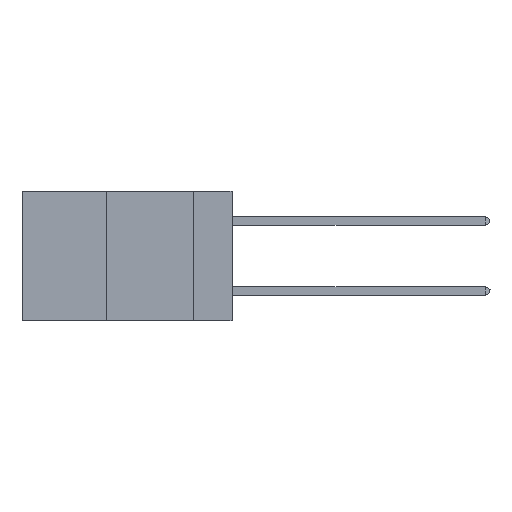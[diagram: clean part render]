
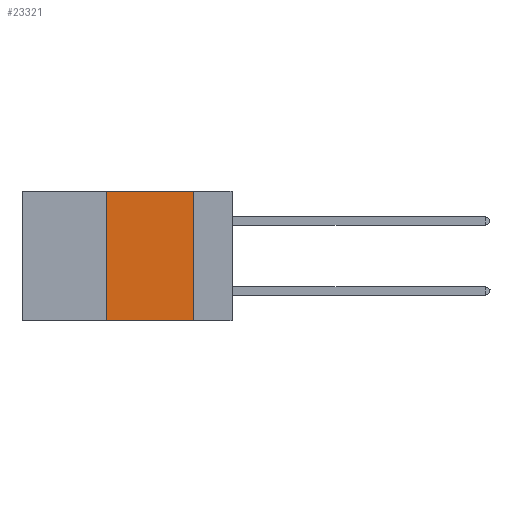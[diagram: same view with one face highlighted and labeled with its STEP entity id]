
A CAD part, left-side view. The second image highlights one B-rep face of the part: STEP entity #23321.
In plain terms, the highlighted planar face has unit normal (-1, 0, 0).
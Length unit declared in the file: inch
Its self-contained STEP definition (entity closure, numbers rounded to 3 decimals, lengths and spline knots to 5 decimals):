
#140 = LINE ( 'NONE', #17243, #11404 ) ;
#777 = VERTEX_POINT ( 'NONE', #6606 ) ;
#1264 = EDGE_CURVE ( 'NONE', #13597, #777, #17549, .T. ) ;
#2304 = CARTESIAN_POINT ( 'NONE',  ( 0., 0.6, 0. ) ) ;
#2401 = VECTOR ( 'NONE', #27061, 39.37008 ) ;
#3879 = DIRECTION ( 'NONE',  ( 0., 0., -1. ) ) ;
#5301 = ORIENTED_EDGE ( 'NONE', *, *, #15979, .F. ) ;
#6434 = ORIENTED_EDGE ( 'NONE', *, *, #1264, .F. ) ;
#6606 = CARTESIAN_POINT ( 'NONE',  ( 0., 0.11, 0. ) ) ;
#6941 = CARTESIAN_POINT ( 'NONE',  ( 0., 0.11, 0. ) ) ;
#9775 = VECTOR ( 'NONE', #18053, 39.37008 ) ;
#10279 = CARTESIAN_POINT ( 'NONE',  ( 0., 0.36, -0.37 ) ) ;
#10882 = EDGE_LOOP ( 'NONE', ( #20947, #6434, #5301, #17719 ) ) ;
#11286 = CARTESIAN_POINT ( 'NONE',  ( 0., 0.6, 0. ) ) ;
#11404 = VECTOR ( 'NONE', #17380, 39.37008 ) ;
#13597 = VERTEX_POINT ( 'NONE', #28049 ) ;
#15979 = EDGE_CURVE ( 'NONE', #26301, #13597, #140, .T. ) ;
#16485 = VERTEX_POINT ( 'NONE', #24046 ) ;
#17138 = PLANE ( 'NONE',  #22886 ) ;
#17243 = CARTESIAN_POINT ( 'NONE',  ( 0., 0.36, 0. ) ) ;
#17380 = DIRECTION ( 'NONE',  ( 0., 0., 1. ) ) ;
#17549 = LINE ( 'NONE', #11286, #25245 ) ;
#17559 = FACE_OUTER_BOUND ( 'NONE', #10882, .T. ) ;
#17719 = ORIENTED_EDGE ( 'NONE', *, *, #24044, .T. ) ;
#18053 = DIRECTION ( 'NONE',  ( 0., 0., -1. ) ) ;
#18365 = CARTESIAN_POINT ( 'NONE',  ( 0., 0.6, -0.37 ) ) ;
#20947 = ORIENTED_EDGE ( 'NONE', *, *, #21210, .F. ) ;
#21210 = EDGE_CURVE ( 'NONE', #777, #16485, #26892, .T. ) ;
#21844 = DIRECTION ( 'NONE',  ( 0., -1., 0. ) ) ;
#22886 = AXIS2_PLACEMENT_3D ( 'NONE', #2304, #27831, #3879 ) ;
#23321 = ADVANCED_FACE ( 'NONE', ( #17559 ), #17138, .F. ) ;
#24044 = EDGE_CURVE ( 'NONE', #26301, #16485, #26930, .T. ) ;
#24046 = CARTESIAN_POINT ( 'NONE',  ( 0., 0.11, -0.37 ) ) ;
#25245 = VECTOR ( 'NONE', #21844, 39.37008 ) ;
#26301 = VERTEX_POINT ( 'NONE', #10279 ) ;
#26892 = LINE ( 'NONE', #6941, #9775 ) ;
#26930 = LINE ( 'NONE', #18365, #2401 ) ;
#27061 = DIRECTION ( 'NONE',  ( 0., -1., 0. ) ) ;
#27831 = DIRECTION ( 'NONE',  ( 1., 0., 0. ) ) ;
#28049 = CARTESIAN_POINT ( 'NONE',  ( 0., 0.36, 0. ) ) ;
